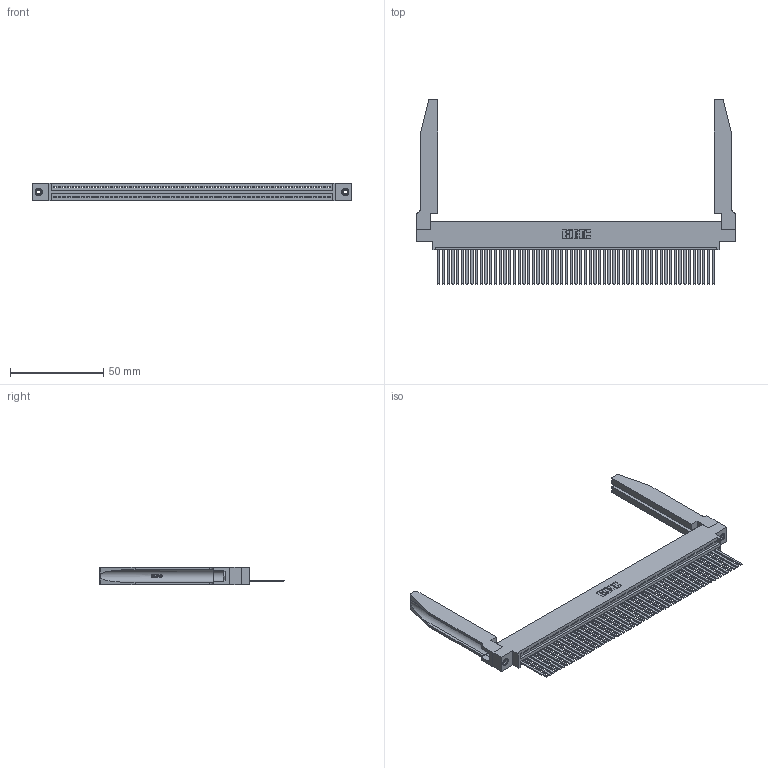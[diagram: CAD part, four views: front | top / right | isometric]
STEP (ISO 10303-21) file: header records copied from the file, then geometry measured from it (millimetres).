
FILE_DESCRIPTION (( 'STEP AP203' ), '1' );
FILE_NAME ('395-059-544-678.STEP', '2019-10-24T10:37:05', ( '' ), ( '' ), 'SwSTEP 2.0', 'SolidWorks 2016', '' );
FILE_SCHEMA (( 'CONFIG_CONTROL_DESIGN' ));
Length unit declared in the file: inch
Products named in the file (5): 395-059-544-678; 345-250-001_345-250-001-102; 345-220-078_345-220-078; 345 Part_0.170 Offset - 0.156 Dia-TH; 345-292-001_345-293-144
Assembly tree (64 placements, depth 2):
  395-059-544-678
    345 Part_0.170 Offset - 0.156 Dia-TH
    345-292-001_345-293-144  x59
    345-250-001_345-250-001-102  x2
    345-220-078_345-220-078  x2
Bounding box: 171.09 x 99.24 x 9.4 mm (x, y, z)
Volume: 24730.4 mm3; surface area: 31792.7 mm2
Topology: 64 solids, 64 shells, 3432 faces, 10283 edges, 6766 vertices
Faces by surface type: plane 2350, cylinder 1030, bspline 36, cone 12, torus 4
Entity records: 46804 total; most frequent: CARTESIAN_POINT 9004, ORIENTED_EDGE 7894, DIRECTION 6843, EDGE_CURVE 3947, LINE 3489, VECTOR 3489, VERTEX_POINT 2624, AXIS2_PLACEMENT_3D 1677
